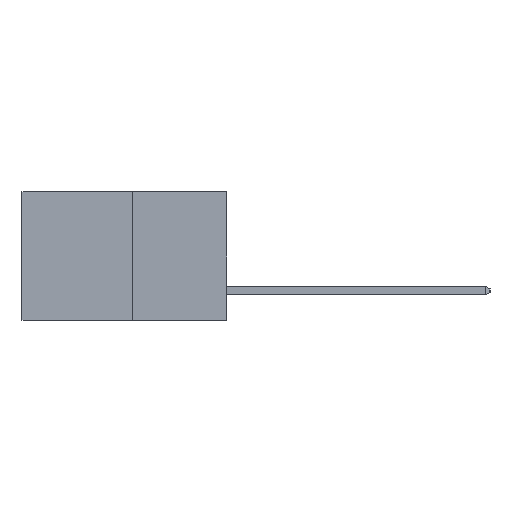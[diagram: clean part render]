
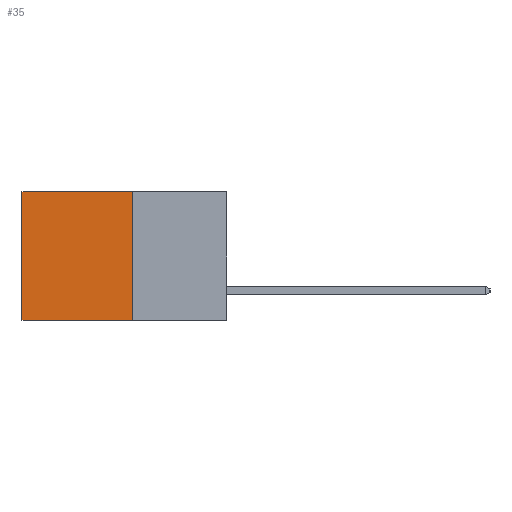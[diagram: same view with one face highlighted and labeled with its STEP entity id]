
A CAD part, left-side view. The second image highlights one B-rep face of the part: STEP entity #35.
In plain terms, the highlighted planar face has unit normal (-1, 0, 0).
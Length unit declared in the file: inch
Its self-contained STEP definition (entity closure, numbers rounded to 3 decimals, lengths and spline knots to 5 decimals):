
#34 = VERTEX_POINT ( 'NONE', #8229 ) ;
#35 = ADVANCED_FACE ( 'NONE', ( #9059 ), #7233, .F. ) ;
#182 = CARTESIAN_POINT ( 'NONE',  ( 0.277, 0.27, 0. ) ) ;
#1107 = VECTOR ( 'NONE', #8317, 39.37008 ) ;
#1138 = VERTEX_POINT ( 'NONE', #182 ) ;
#1644 = ORIENTED_EDGE ( 'NONE', *, *, #4803, .T. ) ;
#2177 = EDGE_LOOP ( 'NONE', ( #1644, #7702, #8958, #5085 ) ) ;
#2331 = VECTOR ( 'NONE', #5712, 39.37008 ) ;
#3209 = VECTOR ( 'NONE', #8713, 39.37008 ) ;
#3712 = VERTEX_POINT ( 'NONE', #8269 ) ;
#4516 = EDGE_CURVE ( 'NONE', #1138, #34, #9709, .T. ) ;
#4803 = EDGE_CURVE ( 'NONE', #7843, #3712, #7217, .T. ) ;
#4820 = EDGE_CURVE ( 'NONE', #1138, #7843, #8935, .T. ) ;
#5085 = ORIENTED_EDGE ( 'NONE', *, *, #4820, .T. ) ;
#5712 = DIRECTION ( 'NONE',  ( 0., 1., 0. ) ) ;
#5731 = CARTESIAN_POINT ( 'NONE',  ( 0.277, 0.27, -0.37 ) ) ;
#6339 = LINE ( 'NONE', #5731, #2331 ) ;
#7125 = CARTESIAN_POINT ( 'NONE',  ( 0.277, 0.59, 0. ) ) ;
#7141 = AXIS2_PLACEMENT_3D ( 'NONE', #7424, #7427, #7413 ) ;
#7217 = LINE ( 'NONE', #8680, #3209 ) ;
#7233 = PLANE ( 'NONE',  #7141 ) ;
#7413 = DIRECTION ( 'NONE',  ( 0., 0., -1. ) ) ;
#7424 = CARTESIAN_POINT ( 'NONE',  ( 0.277, 0.27, -0.37 ) ) ;
#7427 = DIRECTION ( 'NONE',  ( 1., 0., 0. ) ) ;
#7702 = ORIENTED_EDGE ( 'NONE', *, *, #7996, .F. ) ;
#7794 = VECTOR ( 'NONE', #9449, 39.37008 ) ;
#7843 = VERTEX_POINT ( 'NONE', #7125 ) ;
#7996 = EDGE_CURVE ( 'NONE', #34, #3712, #6339, .T. ) ;
#8229 = CARTESIAN_POINT ( 'NONE',  ( 0.277, 0.27, -0.37 ) ) ;
#8269 = CARTESIAN_POINT ( 'NONE',  ( 0.277, 0.59, -0.37 ) ) ;
#8317 = DIRECTION ( 'NONE',  ( 0., 1., 0. ) ) ;
#8362 = CARTESIAN_POINT ( 'NONE',  ( 0.277, 0.27, 0. ) ) ;
#8680 = CARTESIAN_POINT ( 'NONE',  ( 0.277, 0.59, -0.37 ) ) ;
#8713 = DIRECTION ( 'NONE',  ( 0., 0., -1. ) ) ;
#8935 = LINE ( 'NONE', #8362, #1107 ) ;
#8958 = ORIENTED_EDGE ( 'NONE', *, *, #4516, .F. ) ;
#9059 = FACE_OUTER_BOUND ( 'NONE', #2177, .T. ) ;
#9284 = CARTESIAN_POINT ( 'NONE',  ( 0.277, 0.27, -0.37 ) ) ;
#9449 = DIRECTION ( 'NONE',  ( 0., 0., -1. ) ) ;
#9709 = LINE ( 'NONE', #9284, #7794 ) ;
